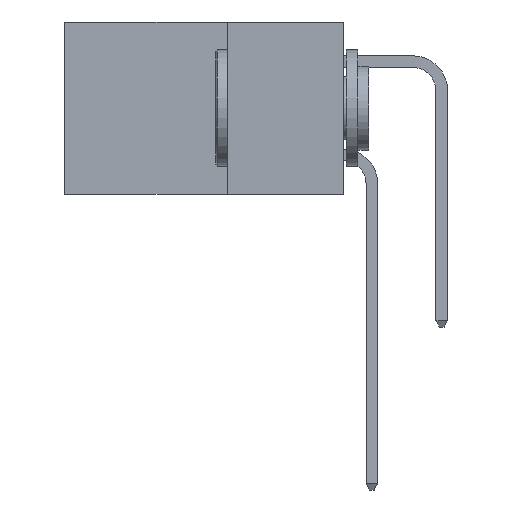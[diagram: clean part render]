
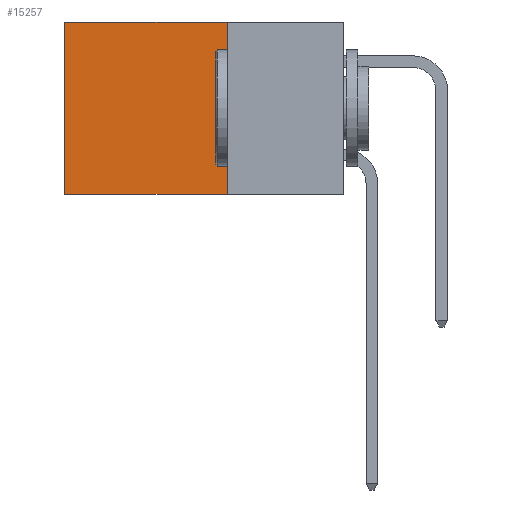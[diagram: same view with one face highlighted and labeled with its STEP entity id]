
A CAD part, left-side view. The second image highlights one B-rep face of the part: STEP entity #15257.
In plain terms, the highlighted planar face has unit normal (-1, 0, 0).
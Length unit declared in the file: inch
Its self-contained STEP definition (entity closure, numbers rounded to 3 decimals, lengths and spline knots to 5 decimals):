
#202 = ORIENTED_EDGE ( 'NONE', *, *, #6166, .T. ) ;
#690 = DIRECTION ( 'NONE',  ( 0., 0., -1. ) ) ;
#1623 = DIRECTION ( 'NONE',  ( 0., 1., 0. ) ) ;
#2402 = CARTESIAN_POINT ( 'NONE',  ( 0.2615, 0.6, -0.37 ) ) ;
#3352 = VECTOR ( 'NONE', #14423, 39.37008 ) ;
#5606 = VECTOR ( 'NONE', #15418, 39.37008 ) ;
#5669 = VERTEX_POINT ( 'NONE', #9656 ) ;
#6166 = EDGE_CURVE ( 'NONE', #12493, #5669, #19842, .T. ) ;
#6694 = CARTESIAN_POINT ( 'NONE',  ( 0.2615, 0.25, -0.37 ) ) ;
#6889 = EDGE_LOOP ( 'NONE', ( #8000, #8479, #14721, #202 ) ) ;
#7112 = PLANE ( 'NONE',  #19798 ) ;
#8000 = ORIENTED_EDGE ( 'NONE', *, *, #16585, .T. ) ;
#8479 = ORIENTED_EDGE ( 'NONE', *, *, #15584, .F. ) ;
#8681 = CARTESIAN_POINT ( 'NONE',  ( 0.2615, 0.25, -0.37 ) ) ;
#9551 = CARTESIAN_POINT ( 'NONE',  ( 0.2615, 0.6, -0.37 ) ) ;
#9656 = CARTESIAN_POINT ( 'NONE',  ( 0.2615, 0.6, 0. ) ) ;
#9957 = VECTOR ( 'NONE', #16379, 39.37008 ) ;
#10257 = DIRECTION ( 'NONE',  ( 1., 0., 0. ) ) ;
#11727 = VERTEX_POINT ( 'NONE', #9551 ) ;
#12493 = VERTEX_POINT ( 'NONE', #14551 ) ;
#13896 = CARTESIAN_POINT ( 'NONE',  ( 0.2615, 0.25, -0.37 ) ) ;
#14423 = DIRECTION ( 'NONE',  ( 0., 0., -1. ) ) ;
#14551 = CARTESIAN_POINT ( 'NONE',  ( 0.2615, 0.25, 0. ) ) ;
#14656 = VERTEX_POINT ( 'NONE', #18124 ) ;
#14721 = ORIENTED_EDGE ( 'NONE', *, *, #16382, .F. ) ;
#14939 = VECTOR ( 'NONE', #1623, 39.37008 ) ;
#15257 = ADVANCED_FACE ( 'NONE', ( #16480 ), #7112, .F. ) ;
#15418 = DIRECTION ( 'NONE',  ( 0., 1., 0. ) ) ;
#15584 = EDGE_CURVE ( 'NONE', #14656, #11727, #17879, .T. ) ;
#15594 = CARTESIAN_POINT ( 'NONE',  ( 0.2615, 0.25, 0. ) ) ;
#16203 = LINE ( 'NONE', #6694, #3352 ) ;
#16379 = DIRECTION ( 'NONE',  ( 0., 0., -1. ) ) ;
#16382 = EDGE_CURVE ( 'NONE', #12493, #14656, #16203, .T. ) ;
#16480 = FACE_OUTER_BOUND ( 'NONE', #6889, .T. ) ;
#16585 = EDGE_CURVE ( 'NONE', #5669, #11727, #18051, .T. ) ;
#17879 = LINE ( 'NONE', #13896, #5606 ) ;
#18051 = LINE ( 'NONE', #2402, #9957 ) ;
#18124 = CARTESIAN_POINT ( 'NONE',  ( 0.2615, 0.25, -0.37 ) ) ;
#19798 = AXIS2_PLACEMENT_3D ( 'NONE', #8681, #10257, #690 ) ;
#19842 = LINE ( 'NONE', #15594, #14939 ) ;
